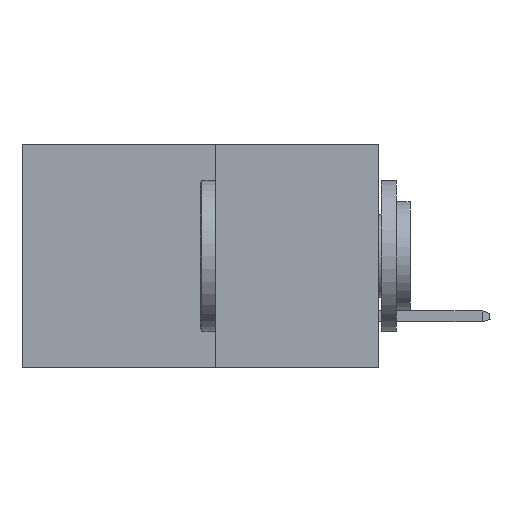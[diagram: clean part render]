
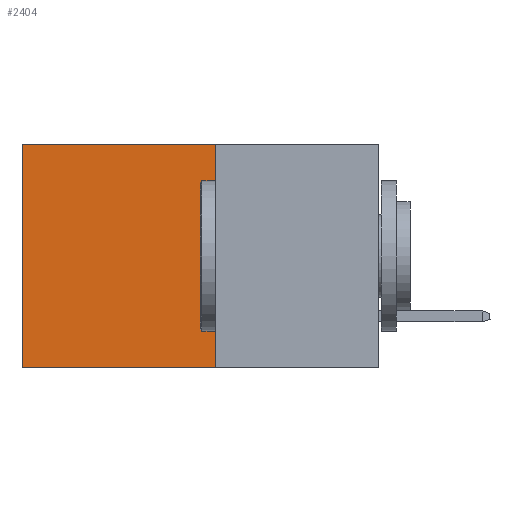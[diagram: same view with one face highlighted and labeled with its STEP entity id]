
A CAD part, left-side view. The second image highlights one B-rep face of the part: STEP entity #2404.
In plain terms, the highlighted planar face has unit normal (-1, 0, 0).
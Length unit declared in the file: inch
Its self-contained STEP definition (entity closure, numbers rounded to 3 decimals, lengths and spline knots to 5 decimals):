
#95 = LINE ( 'NONE', #6425, #11854 ) ;
#530 = CARTESIAN_POINT ( 'NONE',  ( 0.277, 0.27, 0. ) ) ;
#648 = ORIENTED_EDGE ( 'NONE', *, *, #8875, .T. ) ;
#914 = VECTOR ( 'NONE', #6131, 39.37008 ) ;
#1413 = EDGE_CURVE ( 'NONE', #6410, #11536, #7438, .T. ) ;
#2063 = AXIS2_PLACEMENT_3D ( 'NONE', #11310, #10762, #9442 ) ;
#2404 = ADVANCED_FACE ( 'NONE', ( #9053 ), #4693, .F. ) ;
#2538 = CARTESIAN_POINT ( 'NONE',  ( 0.277, 0.59, -0.37 ) ) ;
#2627 = EDGE_CURVE ( 'NONE', #6410, #7909, #3771, .T. ) ;
#3451 = CARTESIAN_POINT ( 'NONE',  ( 0.277, 0.59, -0.37 ) ) ;
#3670 = EDGE_LOOP ( 'NONE', ( #648, #5729, #6389, #9373 ) ) ;
#3771 = LINE ( 'NONE', #9900, #914 ) ;
#4104 = VECTOR ( 'NONE', #11000, 39.37008 ) ;
#4693 = PLANE ( 'NONE',  #2063 ) ;
#4835 = VECTOR ( 'NONE', #12009, 39.37008 ) ;
#5729 = ORIENTED_EDGE ( 'NONE', *, *, #12290, .F. ) ;
#6131 = DIRECTION ( 'NONE',  ( 0., 0., -1. ) ) ;
#6389 = ORIENTED_EDGE ( 'NONE', *, *, #2627, .F. ) ;
#6410 = VERTEX_POINT ( 'NONE', #530 ) ;
#6425 = CARTESIAN_POINT ( 'NONE',  ( 0.277, 0.27, -0.37 ) ) ;
#6661 = LINE ( 'NONE', #3451, #4104 ) ;
#7438 = LINE ( 'NONE', #10294, #4835 ) ;
#7909 = VERTEX_POINT ( 'NONE', #12261 ) ;
#8875 = EDGE_CURVE ( 'NONE', #11536, #9532, #6661, .T. ) ;
#9053 = FACE_OUTER_BOUND ( 'NONE', #3670, .T. ) ;
#9373 = ORIENTED_EDGE ( 'NONE', *, *, #1413, .T. ) ;
#9442 = DIRECTION ( 'NONE',  ( 0., 0., -1. ) ) ;
#9532 = VERTEX_POINT ( 'NONE', #2538 ) ;
#9900 = CARTESIAN_POINT ( 'NONE',  ( 0.277, 0.27, -0.37 ) ) ;
#10294 = CARTESIAN_POINT ( 'NONE',  ( 0.277, 0.27, 0. ) ) ;
#10762 = DIRECTION ( 'NONE',  ( 1., 0., 0. ) ) ;
#11000 = DIRECTION ( 'NONE',  ( 0., 0., -1. ) ) ;
#11137 = DIRECTION ( 'NONE',  ( 0., 1., 0. ) ) ;
#11310 = CARTESIAN_POINT ( 'NONE',  ( 0.277, 0.27, -0.37 ) ) ;
#11536 = VERTEX_POINT ( 'NONE', #11886 ) ;
#11854 = VECTOR ( 'NONE', #11137, 39.37008 ) ;
#11886 = CARTESIAN_POINT ( 'NONE',  ( 0.277, 0.59, 0. ) ) ;
#12009 = DIRECTION ( 'NONE',  ( 0., 1., 0. ) ) ;
#12261 = CARTESIAN_POINT ( 'NONE',  ( 0.277, 0.27, -0.37 ) ) ;
#12290 = EDGE_CURVE ( 'NONE', #7909, #9532, #95, .T. ) ;
